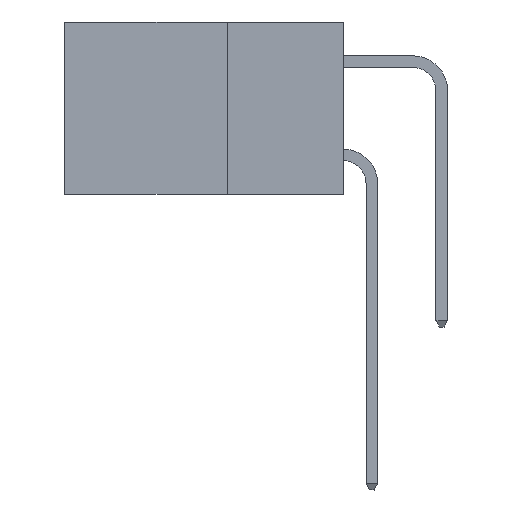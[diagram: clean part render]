
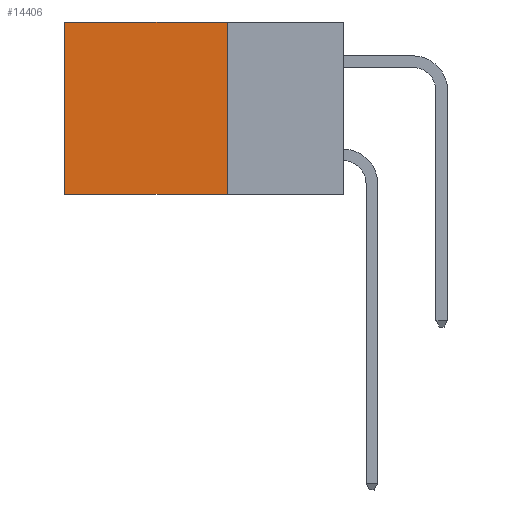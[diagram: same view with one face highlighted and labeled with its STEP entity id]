
A CAD part, left-side view. The second image highlights one B-rep face of the part: STEP entity #14406.
In plain terms, the highlighted planar face has unit normal (-1, 0, 0).
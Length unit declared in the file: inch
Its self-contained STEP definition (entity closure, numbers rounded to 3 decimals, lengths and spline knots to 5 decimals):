
#596 = CARTESIAN_POINT ( 'NONE',  ( 0.298, 0.6, 0. ) ) ;
#654 = FACE_OUTER_BOUND ( 'NONE', #9065, .T. ) ;
#1144 = DIRECTION ( 'NONE',  ( 0., 1., 0. ) ) ;
#1262 = EDGE_CURVE ( 'NONE', #16237, #1387, #15530, .T. ) ;
#1387 = VERTEX_POINT ( 'NONE', #3626 ) ;
#1505 = VECTOR ( 'NONE', #1144, 39.37008 ) ;
#2191 = CARTESIAN_POINT ( 'NONE',  ( 0.298, 0.25, 0. ) ) ;
#2824 = AXIS2_PLACEMENT_3D ( 'NONE', #17067, #6917, #6841 ) ;
#3218 = CARTESIAN_POINT ( 'NONE',  ( 0.298, 0.25, 0. ) ) ;
#3415 = PLANE ( 'NONE',  #2824 ) ;
#3626 = CARTESIAN_POINT ( 'NONE',  ( 0.298, 0.25, -0.37 ) ) ;
#4047 = EDGE_CURVE ( 'NONE', #16659, #12126, #19010, .T. ) ;
#4847 = DIRECTION ( 'NONE',  ( 0., 1., 0. ) ) ;
#6276 = CARTESIAN_POINT ( 'NONE',  ( 0.298, 0.25, -0.37 ) ) ;
#6841 = DIRECTION ( 'NONE',  ( 0., 0., -1. ) ) ;
#6917 = DIRECTION ( 'NONE',  ( 1., 0., 0. ) ) ;
#7014 = ORIENTED_EDGE ( 'NONE', *, *, #1262, .F. ) ;
#7836 = VECTOR ( 'NONE', #11085, 39.37008 ) ;
#8734 = LINE ( 'NONE', #6276, #1505 ) ;
#9065 = EDGE_LOOP ( 'NONE', ( #14977, #17989, #7014, #15746 ) ) ;
#9677 = VECTOR ( 'NONE', #16043, 39.37008 ) ;
#11085 = DIRECTION ( 'NONE',  ( 0., 0., -1. ) ) ;
#12126 = VERTEX_POINT ( 'NONE', #19721 ) ;
#13103 = VECTOR ( 'NONE', #4847, 39.37008 ) ;
#13407 = CARTESIAN_POINT ( 'NONE',  ( 0.298, 0.6, 0. ) ) ;
#13914 = LINE ( 'NONE', #3218, #13103 ) ;
#14406 = ADVANCED_FACE ( 'NONE', ( #654 ), #3415, .F. ) ;
#14977 = ORIENTED_EDGE ( 'NONE', *, *, #4047, .T. ) ;
#15530 = LINE ( 'NONE', #17702, #9677 ) ;
#15746 = ORIENTED_EDGE ( 'NONE', *, *, #16671, .T. ) ;
#16043 = DIRECTION ( 'NONE',  ( 0., 0., -1. ) ) ;
#16237 = VERTEX_POINT ( 'NONE', #2191 ) ;
#16659 = VERTEX_POINT ( 'NONE', #13407 ) ;
#16671 = EDGE_CURVE ( 'NONE', #16237, #16659, #13914, .T. ) ;
#17067 = CARTESIAN_POINT ( 'NONE',  ( 0.298, 0.25, 0. ) ) ;
#17702 = CARTESIAN_POINT ( 'NONE',  ( 0.298, 0.25, 0. ) ) ;
#17989 = ORIENTED_EDGE ( 'NONE', *, *, #21520, .F. ) ;
#19010 = LINE ( 'NONE', #596, #7836 ) ;
#19721 = CARTESIAN_POINT ( 'NONE',  ( 0.298, 0.6, -0.37 ) ) ;
#21520 = EDGE_CURVE ( 'NONE', #1387, #12126, #8734, .T. ) ;
